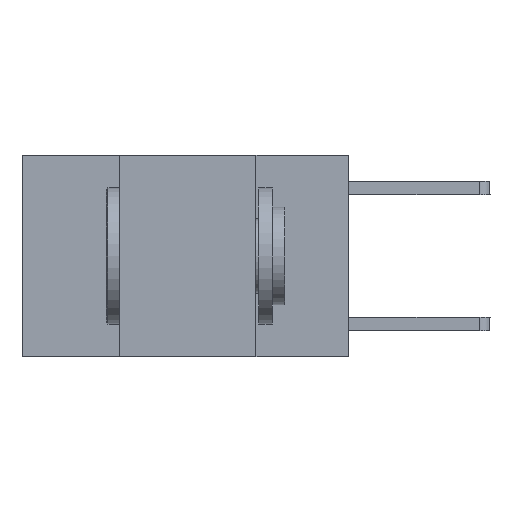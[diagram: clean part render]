
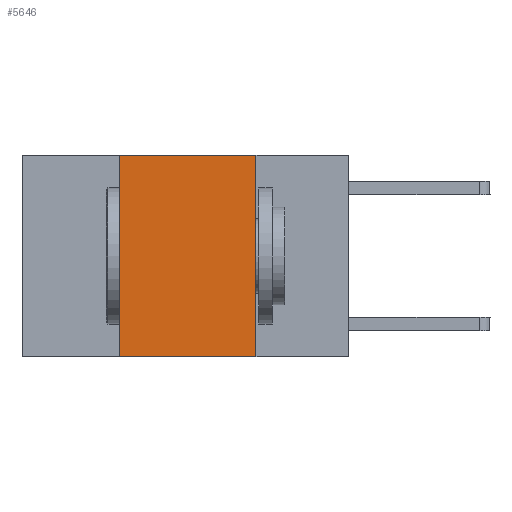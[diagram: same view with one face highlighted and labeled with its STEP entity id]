
A CAD part, left-side view. The second image highlights one B-rep face of the part: STEP entity #5646.
In plain terms, the highlighted planar face has unit normal (-1, 0, 0).
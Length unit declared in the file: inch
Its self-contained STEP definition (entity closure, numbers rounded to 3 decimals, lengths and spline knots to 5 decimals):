
#85 = CARTESIAN_POINT ( 'NONE',  ( 0., 0.17, -0.37 ) ) ;
#1122 = CARTESIAN_POINT ( 'NONE',  ( 0., 0.17, 0. ) ) ;
#1161 = EDGE_CURVE ( 'NONE', #9885, #1810, #3311, .T. ) ;
#1586 = CARTESIAN_POINT ( 'NONE',  ( 0., 0.6, 0. ) ) ;
#1627 = VECTOR ( 'NONE', #8356, 39.37008 ) ;
#1810 = VERTEX_POINT ( 'NONE', #1122 ) ;
#2108 = VERTEX_POINT ( 'NONE', #9177 ) ;
#2221 = EDGE_CURVE ( 'NONE', #2108, #9885, #3812, .T. ) ;
#2542 = DIRECTION ( 'NONE',  ( 0., 0., -1. ) ) ;
#3311 = LINE ( 'NONE', #9320, #1627 ) ;
#3346 = LINE ( 'NONE', #6560, #6067 ) ;
#3420 = DIRECTION ( 'NONE',  ( 1., 0., 0. ) ) ;
#3528 = ORIENTED_EDGE ( 'NONE', *, *, #4783, .F. ) ;
#3812 = LINE ( 'NONE', #6140, #7051 ) ;
#4177 = DIRECTION ( 'NONE',  ( 0., -1., 0. ) ) ;
#4276 = LINE ( 'NONE', #6099, #7730 ) ;
#4432 = DIRECTION ( 'NONE',  ( 0., 0., 1. ) ) ;
#4586 = EDGE_LOOP ( 'NONE', ( #3528, #6328, #10598, #10578 ) ) ;
#4783 = EDGE_CURVE ( 'NONE', #1810, #7596, #4276, .T. ) ;
#5646 = ADVANCED_FACE ( 'NONE', ( #7293 ), #6634, .F. ) ;
#5795 = AXIS2_PLACEMENT_3D ( 'NONE', #1586, #3420, #2542 ) ;
#6067 = VECTOR ( 'NONE', #4177, 39.37008 ) ;
#6099 = CARTESIAN_POINT ( 'NONE',  ( 0., 0.17, 0. ) ) ;
#6140 = CARTESIAN_POINT ( 'NONE',  ( 0., 0.42, 0. ) ) ;
#6328 = ORIENTED_EDGE ( 'NONE', *, *, #1161, .F. ) ;
#6560 = CARTESIAN_POINT ( 'NONE',  ( 0., 0.6, -0.37 ) ) ;
#6634 = PLANE ( 'NONE',  #5795 ) ;
#6871 = DIRECTION ( 'NONE',  ( 0., 0., -1. ) ) ;
#7008 = CARTESIAN_POINT ( 'NONE',  ( 0., 0.42, 0. ) ) ;
#7051 = VECTOR ( 'NONE', #4432, 39.37008 ) ;
#7293 = FACE_OUTER_BOUND ( 'NONE', #4586, .T. ) ;
#7596 = VERTEX_POINT ( 'NONE', #85 ) ;
#7730 = VECTOR ( 'NONE', #6871, 39.37008 ) ;
#8356 = DIRECTION ( 'NONE',  ( 0., -1., 0. ) ) ;
#8769 = EDGE_CURVE ( 'NONE', #2108, #7596, #3346, .T. ) ;
#9177 = CARTESIAN_POINT ( 'NONE',  ( 0., 0.42, -0.37 ) ) ;
#9320 = CARTESIAN_POINT ( 'NONE',  ( 0., 0.6, 0. ) ) ;
#9885 = VERTEX_POINT ( 'NONE', #7008 ) ;
#10578 = ORIENTED_EDGE ( 'NONE', *, *, #8769, .T. ) ;
#10598 = ORIENTED_EDGE ( 'NONE', *, *, #2221, .F. ) ;
